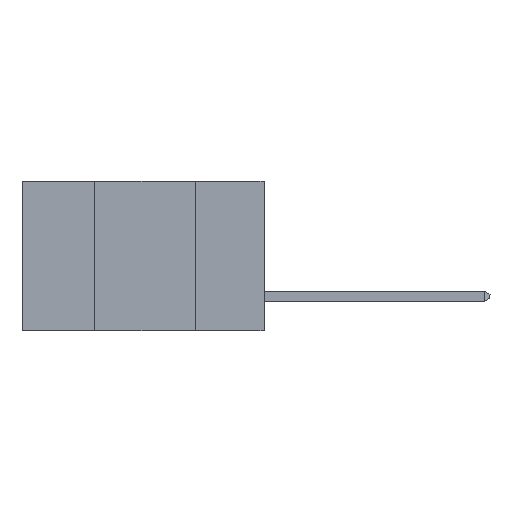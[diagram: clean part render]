
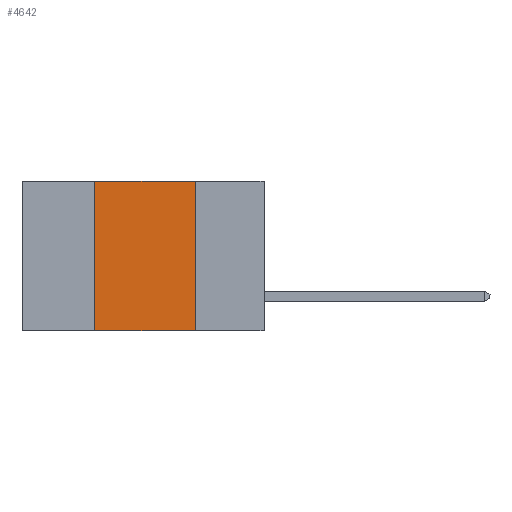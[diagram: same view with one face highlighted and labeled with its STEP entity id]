
A CAD part, left-side view. The second image highlights one B-rep face of the part: STEP entity #4642.
In plain terms, the highlighted planar face has unit normal (-1, 0, 0).
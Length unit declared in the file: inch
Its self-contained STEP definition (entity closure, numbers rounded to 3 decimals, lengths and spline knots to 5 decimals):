
#179 = VECTOR ( 'NONE', #7064, 39.37008 ) ;
#307 = VERTEX_POINT ( 'NONE', #1992 ) ;
#483 = AXIS2_PLACEMENT_3D ( 'NONE', #5702, #5900, #5087 ) ;
#703 = EDGE_LOOP ( 'NONE', ( #931, #3953, #2100, #6755 ) ) ;
#780 = CARTESIAN_POINT ( 'NONE',  ( 0., 0.42, 0. ) ) ;
#858 = LINE ( 'NONE', #6152, #2147 ) ;
#931 = ORIENTED_EDGE ( 'NONE', *, *, #9553, .F. ) ;
#966 = VECTOR ( 'NONE', #5550, 39.37008 ) ;
#1567 = VERTEX_POINT ( 'NONE', #6167 ) ;
#1734 = CARTESIAN_POINT ( 'NONE',  ( 0., 0.6, -0.37 ) ) ;
#1992 = CARTESIAN_POINT ( 'NONE',  ( 0., 0.17, 0. ) ) ;
#2100 = ORIENTED_EDGE ( 'NONE', *, *, #4946, .F. ) ;
#2147 = VECTOR ( 'NONE', #9258, 39.37008 ) ;
#3336 = LINE ( 'NONE', #1734, #179 ) ;
#3387 = VECTOR ( 'NONE', #6957, 39.37008 ) ;
#3889 = CARTESIAN_POINT ( 'NONE',  ( 0., 0.6, 0. ) ) ;
#3953 = ORIENTED_EDGE ( 'NONE', *, *, #5793, .F. ) ;
#4642 = ADVANCED_FACE ( 'NONE', ( #6493 ), #8816, .F. ) ;
#4946 = EDGE_CURVE ( 'NONE', #5224, #5223, #8703, .T. ) ;
#5087 = DIRECTION ( 'NONE',  ( 0., 0., -1. ) ) ;
#5223 = VERTEX_POINT ( 'NONE', #780 ) ;
#5224 = VERTEX_POINT ( 'NONE', #5233 ) ;
#5233 = CARTESIAN_POINT ( 'NONE',  ( 0., 0.42, -0.37 ) ) ;
#5402 = EDGE_CURVE ( 'NONE', #5224, #1567, #3336, .T. ) ;
#5530 = LINE ( 'NONE', #3889, #3387 ) ;
#5550 = DIRECTION ( 'NONE',  ( 0., 0., 1. ) ) ;
#5702 = CARTESIAN_POINT ( 'NONE',  ( 0., 0.6, 0. ) ) ;
#5793 = EDGE_CURVE ( 'NONE', #5223, #307, #5530, .T. ) ;
#5900 = DIRECTION ( 'NONE',  ( 1., 0., 0. ) ) ;
#6152 = CARTESIAN_POINT ( 'NONE',  ( 0., 0.17, -0.37 ) ) ;
#6167 = CARTESIAN_POINT ( 'NONE',  ( 0., 0.17, -0.37 ) ) ;
#6493 = FACE_OUTER_BOUND ( 'NONE', #703, .T. ) ;
#6755 = ORIENTED_EDGE ( 'NONE', *, *, #5402, .T. ) ;
#6957 = DIRECTION ( 'NONE',  ( 0., -1., 0. ) ) ;
#7064 = DIRECTION ( 'NONE',  ( 0., -1., 0. ) ) ;
#8703 = LINE ( 'NONE', #9469, #966 ) ;
#8816 = PLANE ( 'NONE',  #483 ) ;
#9258 = DIRECTION ( 'NONE',  ( 0., 0., -1. ) ) ;
#9469 = CARTESIAN_POINT ( 'NONE',  ( 0., 0.42, -0.37 ) ) ;
#9553 = EDGE_CURVE ( 'NONE', #307, #1567, #858, .T. ) ;
